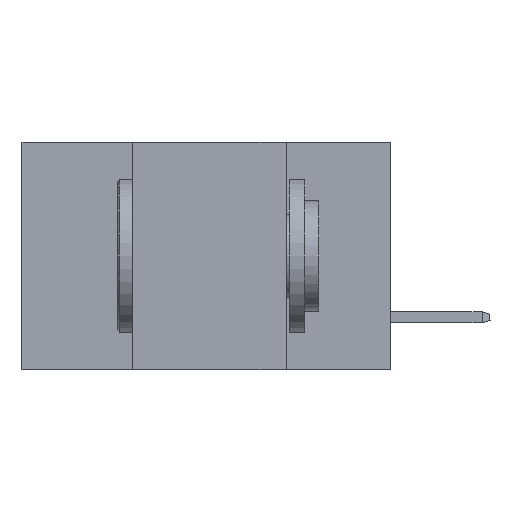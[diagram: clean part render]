
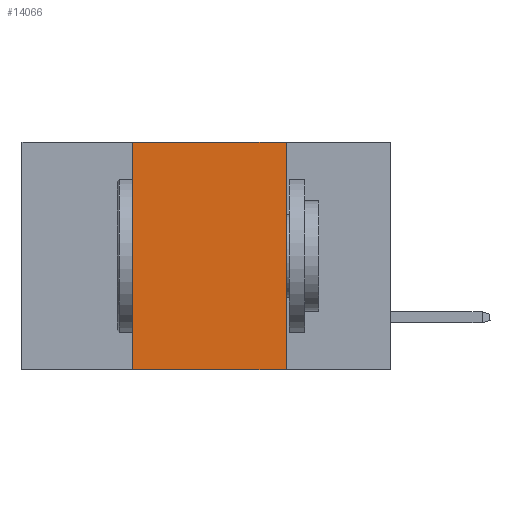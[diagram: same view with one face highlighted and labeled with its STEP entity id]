
A CAD part, left-side view. The second image highlights one B-rep face of the part: STEP entity #14066.
In plain terms, the highlighted planar face has unit normal (-1, 0, 0).
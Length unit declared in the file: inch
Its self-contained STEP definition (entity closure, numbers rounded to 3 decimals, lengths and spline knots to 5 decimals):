
#4 = EDGE_CURVE ( 'NONE', #3369, #13040, #14576, .T. ) ;
#446 = VECTOR ( 'NONE', #18708, 39.37008 ) ;
#735 = PLANE ( 'NONE',  #7384 ) ;
#891 = DIRECTION ( 'NONE',  ( 0., -1., 0. ) ) ;
#1941 = CARTESIAN_POINT ( 'NONE',  ( 0., 0.6, -0.37 ) ) ;
#3369 = VERTEX_POINT ( 'NONE', #10735 ) ;
#3722 = EDGE_CURVE ( 'NONE', #8242, #3369, #7074, .T. ) ;
#3923 = EDGE_CURVE ( 'NONE', #13040, #13991, #12524, .T. ) ;
#4682 = FACE_OUTER_BOUND ( 'NONE', #16403, .T. ) ;
#4836 = ORIENTED_EDGE ( 'NONE', *, *, #4, .F. ) ;
#4945 = VECTOR ( 'NONE', #891, 39.37008 ) ;
#7074 = LINE ( 'NONE', #12717, #16757 ) ;
#7376 = CARTESIAN_POINT ( 'NONE',  ( 0., 0.42, -0.37 ) ) ;
#7384 = AXIS2_PLACEMENT_3D ( 'NONE', #15917, #8327, #17515 ) ;
#7458 = EDGE_CURVE ( 'NONE', #8242, #13991, #18857, .T. ) ;
#8242 = VERTEX_POINT ( 'NONE', #7376 ) ;
#8327 = DIRECTION ( 'NONE',  ( 1., 0., 0. ) ) ;
#9587 = CARTESIAN_POINT ( 'NONE',  ( 0., 0.17, -0.37 ) ) ;
#10735 = CARTESIAN_POINT ( 'NONE',  ( 0., 0.42, 0. ) ) ;
#10826 = ORIENTED_EDGE ( 'NONE', *, *, #3722, .F. ) ;
#11711 = CARTESIAN_POINT ( 'NONE',  ( 0., 0.17, 0. ) ) ;
#12524 = LINE ( 'NONE', #11711, #13684 ) ;
#12717 = CARTESIAN_POINT ( 'NONE',  ( 0., 0.42, 0. ) ) ;
#13011 = CARTESIAN_POINT ( 'NONE',  ( 0., 0.17, 0. ) ) ;
#13040 = VERTEX_POINT ( 'NONE', #13011 ) ;
#13684 = VECTOR ( 'NONE', #13735, 39.37008 ) ;
#13735 = DIRECTION ( 'NONE',  ( 0., 0., -1. ) ) ;
#13960 = CARTESIAN_POINT ( 'NONE',  ( 0., 0.6, 0. ) ) ;
#13991 = VERTEX_POINT ( 'NONE', #9587 ) ;
#14066 = ADVANCED_FACE ( 'NONE', ( #4682 ), #735, .F. ) ;
#14258 = DIRECTION ( 'NONE',  ( 0., 0., 1. ) ) ;
#14576 = LINE ( 'NONE', #13960, #446 ) ;
#15016 = ORIENTED_EDGE ( 'NONE', *, *, #3923, .F. ) ;
#15917 = CARTESIAN_POINT ( 'NONE',  ( 0., 0.6, 0. ) ) ;
#16403 = EDGE_LOOP ( 'NONE', ( #15016, #4836, #10826, #18063 ) ) ;
#16757 = VECTOR ( 'NONE', #14258, 39.37008 ) ;
#17515 = DIRECTION ( 'NONE',  ( 0., 0., -1. ) ) ;
#18063 = ORIENTED_EDGE ( 'NONE', *, *, #7458, .T. ) ;
#18708 = DIRECTION ( 'NONE',  ( 0., -1., 0. ) ) ;
#18857 = LINE ( 'NONE', #1941, #4945 ) ;
